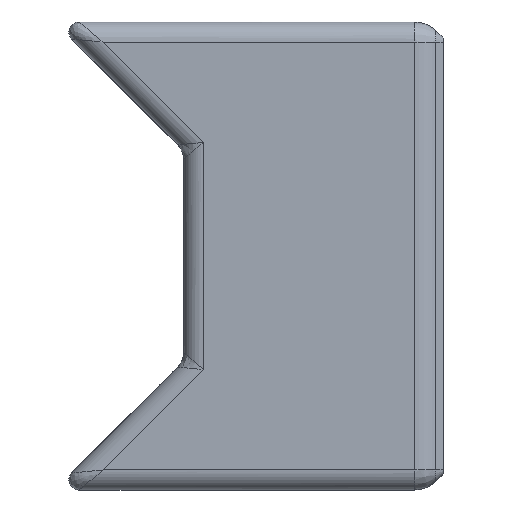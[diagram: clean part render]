
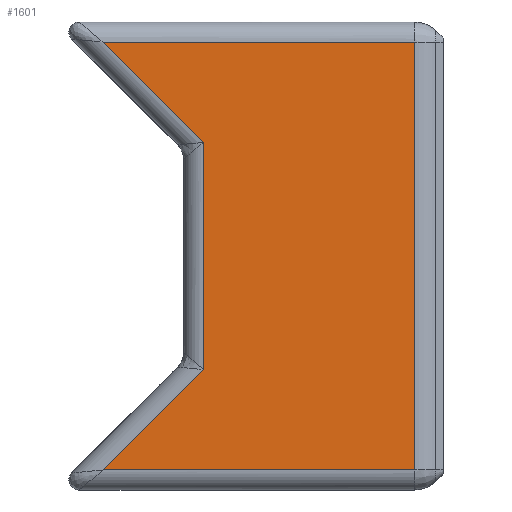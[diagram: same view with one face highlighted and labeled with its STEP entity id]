
A CAD part, left-side view. The second image highlights one B-rep face of the part: STEP entity #1601.
In plain terms, the highlighted planar face has unit normal (-1, 0, 0).
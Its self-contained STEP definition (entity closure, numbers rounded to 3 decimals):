
#123=LINE('',#3068,#197);
#136=LINE('',#3195,#210);
#153=LINE('',#3291,#227);
#154=LINE('',#3295,#228);
#155=LINE('',#3296,#229);
#156=LINE('',#3297,#230);
#197=VECTOR('',#2180,10.);
#210=VECTOR('',#2255,10.);
#227=VECTOR('',#2324,10.);
#228=VECTOR('',#2329,10.);
#229=VECTOR('',#2330,10.);
#230=VECTOR('',#2331,10.);
#298=PLANE('',#1835);
#392=FACE_OUTER_BOUND('',#506,.T.);
#506=EDGE_LOOP('',(#1426,#1427,#1428,#1429,#1430,#1431));
#738=VERTEX_POINT('',#3057);
#740=VERTEX_POINT('',#3067);
#762=VERTEX_POINT('',#3192);
#763=VERTEX_POINT('',#3194);
#780=VERTEX_POINT('',#3290);
#781=VERTEX_POINT('',#3294);
#933=EDGE_CURVE('',#738,#740,#123,.T.);
#967=EDGE_CURVE('',#762,#763,#136,.T.);
#1000=EDGE_CURVE('',#763,#780,#153,.T.);
#1002=EDGE_CURVE('',#781,#762,#154,.T.);
#1003=EDGE_CURVE('',#740,#781,#155,.T.);
#1004=EDGE_CURVE('',#780,#738,#156,.T.);
#1426=ORIENTED_EDGE('',*,*,#967,.F.);
#1427=ORIENTED_EDGE('',*,*,#1002,.F.);
#1428=ORIENTED_EDGE('',*,*,#1003,.F.);
#1429=ORIENTED_EDGE('',*,*,#933,.F.);
#1430=ORIENTED_EDGE('',*,*,#1004,.F.);
#1431=ORIENTED_EDGE('',*,*,#1000,.F.);
#1601=ADVANCED_FACE('',(#392),#298,.F.);
#1835=AXIS2_PLACEMENT_3D('',#3293,#2327,#2328);
#2180=DIRECTION('',(0.,0.,1.));
#2255=DIRECTION('',(0.,0.,-1.));
#2324=DIRECTION('',(0.,1.,0.));
#2327=DIRECTION('center_axis',(1.,0.,0.));
#2328=DIRECTION('ref_axis',(0.,1.,0.));
#2329=DIRECTION('',(0.,-1.,0.));
#2330=DIRECTION('',(0.,0.707,0.707));
#2331=DIRECTION('',(0.,-0.707,0.707));
#3057=CARTESIAN_POINT('',(4.864,-40.769,-133.83));
#3067=CARTESIAN_POINT('',(4.864,-40.769,-128.161));
#3068=CARTESIAN_POINT('',(4.864,-40.769,-128.527));
#3192=CARTESIAN_POINT('',(4.864,-46.039,-125.653));
#3194=CARTESIAN_POINT('',(4.864,-46.039,-136.339));
#3195=CARTESIAN_POINT('',(4.864,-46.039,-129.256));
#3290=CARTESIAN_POINT('',(4.864,-38.26,-136.339));
#3291=CARTESIAN_POINT('',(4.864,-33.864,-136.339));
#3293=CARTESIAN_POINT('Origin',(4.864,-30.459,-128.676));
#3294=CARTESIAN_POINT('',(4.864,-38.26,-125.653));
#3295=CARTESIAN_POINT('',(4.864,-33.864,-125.653));
#3296=CARTESIAN_POINT('',(4.864,-38.071,-125.463));
#3297=CARTESIAN_POINT('',(4.864,-39.231,-135.368));
